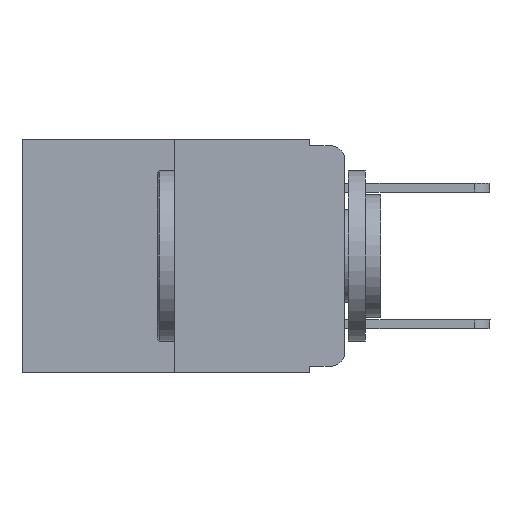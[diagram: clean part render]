
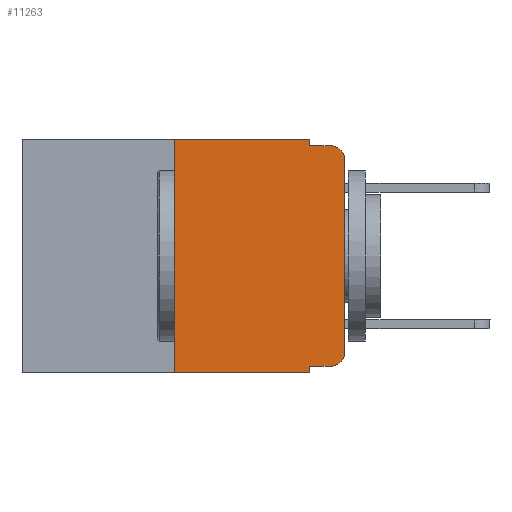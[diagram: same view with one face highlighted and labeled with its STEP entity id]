
A CAD part, left-side view. The second image highlights one B-rep face of the part: STEP entity #11263.
In plain terms, the highlighted planar face has unit normal (-1, 0, 0).
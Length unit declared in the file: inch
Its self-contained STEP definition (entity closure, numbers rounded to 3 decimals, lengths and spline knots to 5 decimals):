
#336 = PLANE ( 'NONE',  #6490 ) ;
#627 = VERTEX_POINT ( 'NONE', #2607 ) ;
#631 = ORIENTED_EDGE ( 'NONE', *, *, #2147, .T. ) ;
#1027 = CARTESIAN_POINT ( 'NONE',  ( 0., 0.051, -0.343 ) ) ;
#1079 = EDGE_CURVE ( 'NONE', #627, #12373, #8839, .T. ) ;
#1263 = VECTOR ( 'NONE', #12700, 39.37008 ) ;
#1731 = VECTOR ( 'NONE', #10573, 39.37008 ) ;
#2103 = ORIENTED_EDGE ( 'NONE', *, *, #3596, .F. ) ;
#2147 = EDGE_CURVE ( 'NONE', #10386, #5619, #12661, .T. ) ;
#2165 = VERTEX_POINT ( 'NONE', #9258 ) ;
#2473 = EDGE_CURVE ( 'NONE', #7369, #2165, #3956, .T. ) ;
#2498 = CARTESIAN_POINT ( 'NONE',  ( 0., 0.25, 0. ) ) ;
#2586 = EDGE_CURVE ( 'NONE', #10713, #7386, #8315, .T. ) ;
#2607 = CARTESIAN_POINT ( 'NONE',  ( 0., 0.25, 0. ) ) ;
#2646 = CARTESIAN_POINT ( 'NONE',  ( 0., 0.051, 0. ) ) ;
#3465 = CARTESIAN_POINT ( 'NONE',  ( 0., 0., -0.03 ) ) ;
#3492 = CARTESIAN_POINT ( 'NONE',  ( 0., 0.02, -0.313 ) ) ;
#3542 = DIRECTION ( 'NONE',  ( -1., 0., 0. ) ) ;
#3596 = EDGE_CURVE ( 'NONE', #4610, #5619, #11115, .T. ) ;
#3642 = CARTESIAN_POINT ( 'NONE',  ( 0., 0.473, -0.343 ) ) ;
#3746 = DIRECTION ( 'NONE',  ( 0., 0., 1. ) ) ;
#3956 = CIRCLE ( 'NONE', #5691, 0.02 ) ;
#4093 = CARTESIAN_POINT ( 'NONE',  ( 0., 0.051, 0. ) ) ;
#4200 = CARTESIAN_POINT ( 'NONE',  ( 0., 0.051, 0. ) ) ;
#4279 = ORIENTED_EDGE ( 'NONE', *, *, #7579, .F. ) ;
#4492 = CARTESIAN_POINT ( 'NONE',  ( 0., 0., 0. ) ) ;
#4610 = VERTEX_POINT ( 'NONE', #6799 ) ;
#4653 = DIRECTION ( 'NONE',  ( 1., 0., 0. ) ) ;
#4671 = CARTESIAN_POINT ( 'NONE',  ( 0., 0.051, -0.01 ) ) ;
#4749 = ORIENTED_EDGE ( 'NONE', *, *, #2586, .T. ) ;
#4837 = EDGE_CURVE ( 'NONE', #4610, #7369, #5068, .T. ) ;
#4965 = LINE ( 'NONE', #9001, #8819 ) ;
#5022 = DIRECTION ( 'NONE',  ( 0., -1., 0. ) ) ;
#5068 = LINE ( 'NONE', #13630, #1731 ) ;
#5233 = CARTESIAN_POINT ( 'NONE',  ( 0., 0.02, -0.333 ) ) ;
#5501 = VECTOR ( 'NONE', #10035, 39.37008 ) ;
#5580 = VECTOR ( 'NONE', #8914, 39.37008 ) ;
#5586 = CARTESIAN_POINT ( 'NONE',  ( 0., 0.473, 0. ) ) ;
#5619 = VERTEX_POINT ( 'NONE', #1027 ) ;
#5684 = LINE ( 'NONE', #2498, #7863 ) ;
#5691 = AXIS2_PLACEMENT_3D ( 'NONE', #3492, #3542, #11016 ) ;
#5699 = EDGE_LOOP ( 'NONE', ( #8339, #4749, #9266, #4279, #12627, #5930, #631, #2103, #11041, #7623 ) ) ;
#5930 = ORIENTED_EDGE ( 'NONE', *, *, #12802, .F. ) ;
#5939 = AXIS2_PLACEMENT_3D ( 'NONE', #10084, #12188, #6927 ) ;
#5968 = LINE ( 'NONE', #2646, #5501 ) ;
#6490 = AXIS2_PLACEMENT_3D ( 'NONE', #5586, #4653, #12115 ) ;
#6799 = CARTESIAN_POINT ( 'NONE',  ( 0., 0.051, -0.333 ) ) ;
#6927 = DIRECTION ( 'NONE',  ( 0., 0., -1. ) ) ;
#7369 = VERTEX_POINT ( 'NONE', #5233 ) ;
#7386 = VERTEX_POINT ( 'NONE', #7389 ) ;
#7389 = CARTESIAN_POINT ( 'NONE',  ( 0., 0.02, -0.01 ) ) ;
#7579 = EDGE_CURVE ( 'NONE', #12373, #10085, #5968, .T. ) ;
#7623 = ORIENTED_EDGE ( 'NONE', *, *, #2473, .T. ) ;
#7716 = FACE_OUTER_BOUND ( 'NONE', #5699, .T. ) ;
#7863 = VECTOR ( 'NONE', #3746, 39.37008 ) ;
#7960 = DIRECTION ( 'NONE',  ( 0., -1., 0. ) ) ;
#8244 = EDGE_CURVE ( 'NONE', #10085, #7386, #4965, .T. ) ;
#8315 = CIRCLE ( 'NONE', #5939, 0.02 ) ;
#8339 = ORIENTED_EDGE ( 'NONE', *, *, #10053, .T. ) ;
#8457 = CARTESIAN_POINT ( 'NONE',  ( 0., 0.473, 0. ) ) ;
#8815 = VECTOR ( 'NONE', #7960, 39.37008 ) ;
#8819 = VECTOR ( 'NONE', #5022, 39.37008 ) ;
#8839 = LINE ( 'NONE', #8457, #11328 ) ;
#8914 = DIRECTION ( 'NONE',  ( 0., 0., 1. ) ) ;
#9001 = CARTESIAN_POINT ( 'NONE',  ( 0., 0.051, -0.01 ) ) ;
#9258 = CARTESIAN_POINT ( 'NONE',  ( 0., 0., -0.313 ) ) ;
#9266 = ORIENTED_EDGE ( 'NONE', *, *, #8244, .F. ) ;
#10035 = DIRECTION ( 'NONE',  ( 0., 0., -1. ) ) ;
#10053 = EDGE_CURVE ( 'NONE', #2165, #10713, #11090, .T. ) ;
#10084 = CARTESIAN_POINT ( 'NONE',  ( 0., 0.02, -0.03 ) ) ;
#10085 = VERTEX_POINT ( 'NONE', #4671 ) ;
#10309 = CARTESIAN_POINT ( 'NONE',  ( 0., 0.25, -0.343 ) ) ;
#10386 = VERTEX_POINT ( 'NONE', #10309 ) ;
#10573 = DIRECTION ( 'NONE',  ( 0., -1., 0. ) ) ;
#10713 = VERTEX_POINT ( 'NONE', #3465 ) ;
#11016 = DIRECTION ( 'NONE',  ( 0., 0., -1. ) ) ;
#11041 = ORIENTED_EDGE ( 'NONE', *, *, #4837, .T. ) ;
#11090 = LINE ( 'NONE', #4492, #5580 ) ;
#11115 = LINE ( 'NONE', #4200, #1263 ) ;
#11263 = ADVANCED_FACE ( 'NONE', ( #7716 ), #336, .F. ) ;
#11328 = VECTOR ( 'NONE', #11622, 39.37008 ) ;
#11622 = DIRECTION ( 'NONE',  ( 0., -1., 0. ) ) ;
#12115 = DIRECTION ( 'NONE',  ( 0., 0., -1. ) ) ;
#12188 = DIRECTION ( 'NONE',  ( -1., 0., 0. ) ) ;
#12373 = VERTEX_POINT ( 'NONE', #4093 ) ;
#12627 = ORIENTED_EDGE ( 'NONE', *, *, #1079, .F. ) ;
#12661 = LINE ( 'NONE', #3642, #8815 ) ;
#12700 = DIRECTION ( 'NONE',  ( 0., 0., -1. ) ) ;
#12802 = EDGE_CURVE ( 'NONE', #10386, #627, #5684, .T. ) ;
#13630 = CARTESIAN_POINT ( 'NONE',  ( 0., 0.051, -0.333 ) ) ;
